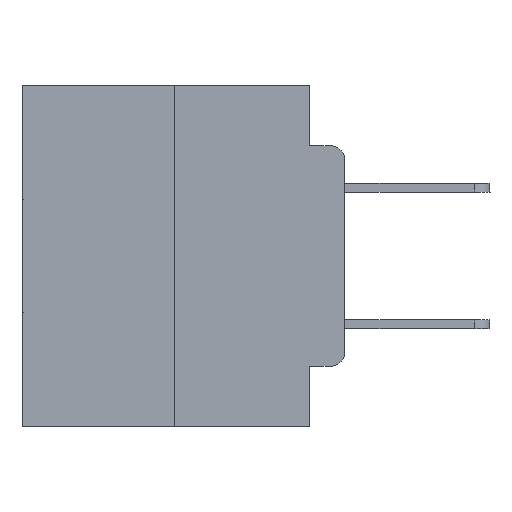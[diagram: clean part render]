
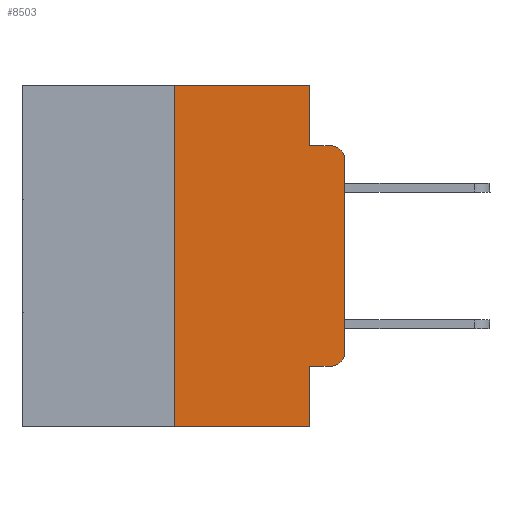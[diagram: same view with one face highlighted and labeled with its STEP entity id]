
A CAD part, left-side view. The second image highlights one B-rep face of the part: STEP entity #8503.
In plain terms, the highlighted planar face has unit normal (-1, 0, 0).
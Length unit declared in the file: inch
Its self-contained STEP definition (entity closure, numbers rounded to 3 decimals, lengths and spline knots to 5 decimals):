
#75 = CARTESIAN_POINT ( 'NONE',  ( 0., 0.051, 0. ) ) ;
#909 = ORIENTED_EDGE ( 'NONE', *, *, #25458, .T. ) ;
#910 = DIRECTION ( 'NONE',  ( 1., 0., 0. ) ) ;
#1755 = VERTEX_POINT ( 'NONE', #25062 ) ;
#2238 = DIRECTION ( 'NONE',  ( -1., 0., 0. ) ) ;
#2395 = VECTOR ( 'NONE', #8516, 39.37008 ) ;
#2532 = CARTESIAN_POINT ( 'NONE',  ( 0., 0.25, -0.5 ) ) ;
#2745 = LINE ( 'NONE', #19455, #2395 ) ;
#2802 = ORIENTED_EDGE ( 'NONE', *, *, #21855, .T. ) ;
#2832 = LINE ( 'NONE', #4939, #20816 ) ;
#3008 = EDGE_CURVE ( 'NONE', #21433, #1755, #13117, .T. ) ;
#3309 = CARTESIAN_POINT ( 'NONE',  ( 0., 0.02, -0.0885 ) ) ;
#3401 = ORIENTED_EDGE ( 'NONE', *, *, #3008, .F. ) ;
#4477 = ORIENTED_EDGE ( 'NONE', *, *, #10827, .T. ) ;
#4891 = VERTEX_POINT ( 'NONE', #8608 ) ;
#4939 = CARTESIAN_POINT ( 'NONE',  ( 0., 0.051, -0.4115 ) ) ;
#5086 = EDGE_CURVE ( 'NONE', #21433, #4891, #2832, .T. ) ;
#5648 = ORIENTED_EDGE ( 'NONE', *, *, #20603, .F. ) ;
#5997 = ORIENTED_EDGE ( 'NONE', *, *, #5086, .T. ) ;
#6237 = VERTEX_POINT ( 'NONE', #20803 ) ;
#6666 = VECTOR ( 'NONE', #12300, 39.37008 ) ;
#6783 = DIRECTION ( 'NONE',  ( 0., 0., -1. ) ) ;
#7342 = PLANE ( 'NONE',  #20588 ) ;
#8503 = ADVANCED_FACE ( 'NONE', ( #20662 ), #7342, .F. ) ;
#8516 = DIRECTION ( 'NONE',  ( 0., 0., 1. ) ) ;
#8608 = CARTESIAN_POINT ( 'NONE',  ( 0., 0.02, -0.4115 ) ) ;
#8733 = DIRECTION ( 'NONE',  ( -1., 0., 0. ) ) ;
#9278 = LINE ( 'NONE', #13568, #23919 ) ;
#9458 = LINE ( 'NONE', #75, #25459 ) ;
#9465 = CARTESIAN_POINT ( 'NONE',  ( 0., 0.051, -0.0885 ) ) ;
#9495 = EDGE_CURVE ( 'NONE', #23118, #14287, #15429, .T. ) ;
#10135 = VECTOR ( 'NONE', #25221, 39.37008 ) ;
#10416 = VERTEX_POINT ( 'NONE', #3309 ) ;
#10827 = EDGE_CURVE ( 'NONE', #4891, #17055, #14288, .T. ) ;
#11058 = DIRECTION ( 'NONE',  ( 0., 0., -1. ) ) ;
#11298 = VECTOR ( 'NONE', #14753, 39.37008 ) ;
#11428 = CARTESIAN_POINT ( 'NONE',  ( 0., 0.473, 0. ) ) ;
#11876 = ORIENTED_EDGE ( 'NONE', *, *, #9495, .F. ) ;
#12050 = VERTEX_POINT ( 'NONE', #9465 ) ;
#12300 = DIRECTION ( 'NONE',  ( 0., 0., -1. ) ) ;
#12558 = CARTESIAN_POINT ( 'NONE',  ( 0., 0.473, 0. ) ) ;
#13117 = LINE ( 'NONE', #25418, #6666 ) ;
#13568 = CARTESIAN_POINT ( 'NONE',  ( 0., 0.473, -0.5 ) ) ;
#13938 = DIRECTION ( 'NONE',  ( 0., -1., 0. ) ) ;
#14099 = CARTESIAN_POINT ( 'NONE',  ( 0., 0.051, -0.0885 ) ) ;
#14287 = VERTEX_POINT ( 'NONE', #28113 ) ;
#14288 = CIRCLE ( 'NONE', #14326, 0.02 ) ;
#14326 = AXIS2_PLACEMENT_3D ( 'NONE', #17394, #2238, #23775 ) ;
#14558 = AXIS2_PLACEMENT_3D ( 'NONE', #15231, #8733, #6783 ) ;
#14561 = LINE ( 'NONE', #14099, #10135 ) ;
#14753 = DIRECTION ( 'NONE',  ( 0., -1., 0. ) ) ;
#15231 = CARTESIAN_POINT ( 'NONE',  ( 0., 0.02, -0.1085 ) ) ;
#15429 = LINE ( 'NONE', #18664, #23558 ) ;
#15997 = ORIENTED_EDGE ( 'NONE', *, *, #26128, .T. ) ;
#16076 = DIRECTION ( 'NONE',  ( 0., 0., -1. ) ) ;
#16726 = EDGE_CURVE ( 'NONE', #25600, #12050, #9458, .T. ) ;
#17055 = VERTEX_POINT ( 'NONE', #27665 ) ;
#17394 = CARTESIAN_POINT ( 'NONE',  ( 0., 0.02, -0.3915 ) ) ;
#17422 = LINE ( 'NONE', #12558, #11298 ) ;
#18664 = CARTESIAN_POINT ( 'NONE',  ( 0., 0.25, 0. ) ) ;
#19083 = EDGE_LOOP ( 'NONE', ( #2802, #909, #23682, #19516, #5648, #11876, #15997, #3401, #5997, #4477 ) ) ;
#19455 = CARTESIAN_POINT ( 'NONE',  ( 0., 0., 0. ) ) ;
#19516 = ORIENTED_EDGE ( 'NONE', *, *, #16726, .F. ) ;
#20588 = AXIS2_PLACEMENT_3D ( 'NONE', #11428, #910, #16076 ) ;
#20603 = EDGE_CURVE ( 'NONE', #14287, #25600, #17422, .T. ) ;
#20662 = FACE_OUTER_BOUND ( 'NONE', #19083, .T. ) ;
#20803 = CARTESIAN_POINT ( 'NONE',  ( 0., 0., -0.1085 ) ) ;
#20816 = VECTOR ( 'NONE', #26778, 39.37008 ) ;
#21433 = VERTEX_POINT ( 'NONE', #26534 ) ;
#21855 = EDGE_CURVE ( 'NONE', #17055, #6237, #2745, .T. ) ;
#23118 = VERTEX_POINT ( 'NONE', #2532 ) ;
#23558 = VECTOR ( 'NONE', #25509, 39.37008 ) ;
#23682 = ORIENTED_EDGE ( 'NONE', *, *, #27744, .F. ) ;
#23775 = DIRECTION ( 'NONE',  ( 0., 0., -1. ) ) ;
#23919 = VECTOR ( 'NONE', #13938, 39.37008 ) ;
#24697 = CARTESIAN_POINT ( 'NONE',  ( 0., 0.051, 0. ) ) ;
#25062 = CARTESIAN_POINT ( 'NONE',  ( 0., 0.051, -0.5 ) ) ;
#25221 = DIRECTION ( 'NONE',  ( 0., -1., 0. ) ) ;
#25418 = CARTESIAN_POINT ( 'NONE',  ( 0., 0.051, 0. ) ) ;
#25458 = EDGE_CURVE ( 'NONE', #6237, #10416, #25594, .T. ) ;
#25459 = VECTOR ( 'NONE', #11058, 39.37008 ) ;
#25509 = DIRECTION ( 'NONE',  ( 0., 0., 1. ) ) ;
#25594 = CIRCLE ( 'NONE', #14558, 0.02 ) ;
#25600 = VERTEX_POINT ( 'NONE', #24697 ) ;
#26128 = EDGE_CURVE ( 'NONE', #23118, #1755, #9278, .T. ) ;
#26534 = CARTESIAN_POINT ( 'NONE',  ( 0., 0.051, -0.4115 ) ) ;
#26778 = DIRECTION ( 'NONE',  ( 0., -1., 0. ) ) ;
#27665 = CARTESIAN_POINT ( 'NONE',  ( 0., 0., -0.3915 ) ) ;
#27744 = EDGE_CURVE ( 'NONE', #12050, #10416, #14561, .T. ) ;
#28113 = CARTESIAN_POINT ( 'NONE',  ( 0., 0.25, 0. ) ) ;
